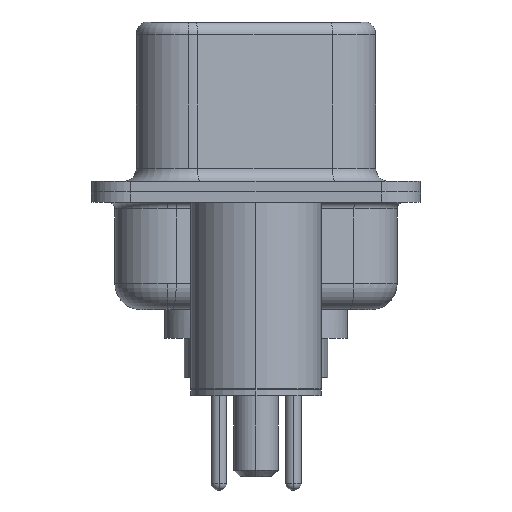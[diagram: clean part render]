
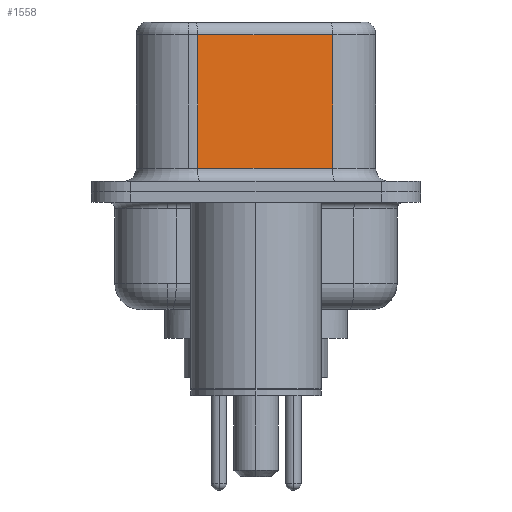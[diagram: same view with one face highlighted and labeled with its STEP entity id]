
A CAD part, left-side view. The second image highlights one B-rep face of the part: STEP entity #1558.
In plain terms, the highlighted planar face has unit normal (-0.985, -0.174, 0).
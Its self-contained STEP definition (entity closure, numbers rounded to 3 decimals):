
#204 = LINE ( 'NONE', #3812, #18095 ) ;
#487 = DIRECTION ( 'NONE',  ( 0.174, -0.985, 0. ) ) ;
#1299 = VERTEX_POINT ( 'NONE', #15263 ) ;
#1558 = ADVANCED_FACE ( 'NONE', ( #2850 ), #4194, .F. ) ;
#1563 = ORIENTED_EDGE ( 'NONE', *, *, #3564, .F. ) ;
#2850 = FACE_OUTER_BOUND ( 'NONE', #10898, .T. ) ;
#2939 = ORIENTED_EDGE ( 'NONE', *, *, #6432, .T. ) ;
#3564 = EDGE_CURVE ( 'NONE', #1299, #12005, #13685, .T. ) ;
#3812 = CARTESIAN_POINT ( 'NONE',  ( 3.67, 2.233, 6.52 ) ) ;
#4194 = PLANE ( 'NONE',  #17729 ) ;
#4313 = DIRECTION ( 'NONE',  ( 0., 0., -1. ) ) ;
#5105 = CARTESIAN_POINT ( 'NONE',  ( 4.58, -2.927, 0.9 ) ) ;
#5219 = DIRECTION ( 'NONE',  ( 0., 0., -1. ) ) ;
#5430 = VECTOR ( 'NONE', #487, 1000. ) ;
#5806 = CARTESIAN_POINT ( 'NONE',  ( 4.58, -2.927, 6.02 ) ) ;
#5867 = VERTEX_POINT ( 'NONE', #9305 ) ;
#6432 = EDGE_CURVE ( 'NONE', #1299, #5867, #9576, .T. ) ;
#7839 = ORIENTED_EDGE ( 'NONE', *, *, #9313, .T. ) ;
#8884 = VERTEX_POINT ( 'NONE', #15205 ) ;
#9284 = LINE ( 'NONE', #17354, #5430 ) ;
#9305 = CARTESIAN_POINT ( 'NONE',  ( 3.67, 2.233, 6.02 ) ) ;
#9313 = EDGE_CURVE ( 'NONE', #8884, #12005, #9284, .T. ) ;
#9576 = LINE ( 'NONE', #5806, #12901 ) ;
#9931 = VECTOR ( 'NONE', #4313, 1000. ) ;
#10018 = DIRECTION ( 'NONE',  ( -0.174, 0.985, 0. ) ) ;
#10898 = EDGE_LOOP ( 'NONE', ( #1563, #2939, #11982, #7839 ) ) ;
#11005 = CARTESIAN_POINT ( 'NONE',  ( 4.58, -2.927, 6.52 ) ) ;
#11982 = ORIENTED_EDGE ( 'NONE', *, *, #17198, .T. ) ;
#12005 = VERTEX_POINT ( 'NONE', #5105 ) ;
#12442 = DIRECTION ( 'NONE',  ( 0.985, 0.174, 0. ) ) ;
#12587 = DIRECTION ( 'NONE',  ( -0.174, 0.985, 0. ) ) ;
#12901 = VECTOR ( 'NONE', #10018, 1000. ) ;
#13685 = LINE ( 'NONE', #17953, #9931 ) ;
#15205 = CARTESIAN_POINT ( 'NONE',  ( 3.67, 2.233, 0.9 ) ) ;
#15263 = CARTESIAN_POINT ( 'NONE',  ( 4.58, -2.927, 6.02 ) ) ;
#17198 = EDGE_CURVE ( 'NONE', #5867, #8884, #204, .T. ) ;
#17354 = CARTESIAN_POINT ( 'NONE',  ( 4.58, -2.927, 0.9 ) ) ;
#17729 = AXIS2_PLACEMENT_3D ( 'NONE', #11005, #12442, #12587 ) ;
#17953 = CARTESIAN_POINT ( 'NONE',  ( 4.58, -2.927, 6.52 ) ) ;
#18095 = VECTOR ( 'NONE', #5219, 1000. ) ;
